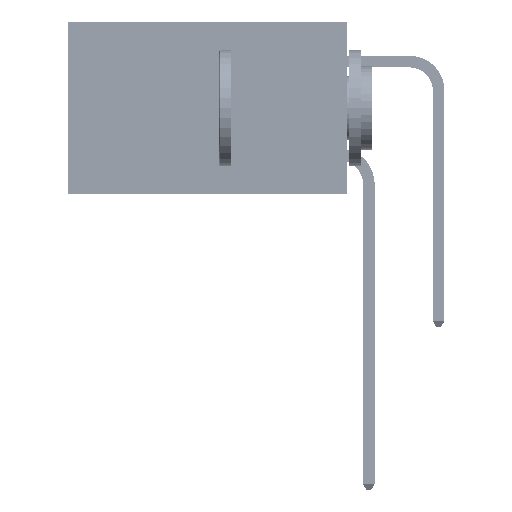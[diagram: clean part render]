
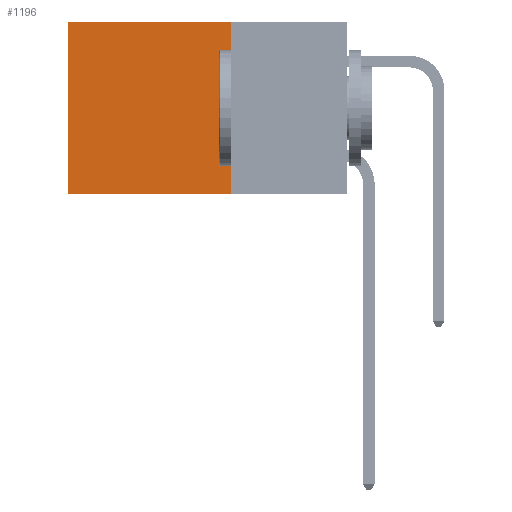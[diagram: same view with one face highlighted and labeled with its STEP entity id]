
A CAD part, left-side view. The second image highlights one B-rep face of the part: STEP entity #1196.
In plain terms, the highlighted planar face has unit normal (-1, 0, 0).
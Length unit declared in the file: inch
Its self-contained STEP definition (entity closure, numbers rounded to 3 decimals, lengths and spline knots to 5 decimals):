
#657 = FACE_OUTER_BOUND ( 'NONE', #15246, .T. ) ;
#1196 = ADVANCED_FACE ( 'NONE', ( #657 ), #12207, .F. ) ;
#1777 = VECTOR ( 'NONE', #40079, 39.37008 ) ;
#3276 = CARTESIAN_POINT ( 'NONE',  ( 0.2875, 0.6, -0.37 ) ) ;
#4918 = CARTESIAN_POINT ( 'NONE',  ( 0.2875, 0.25, 0. ) ) ;
#5480 = ORIENTED_EDGE ( 'NONE', *, *, #32674, .T. ) ;
#9277 = EDGE_CURVE ( 'NONE', #25299, #16981, #23393, .T. ) ;
#10438 = VECTOR ( 'NONE', #32113, 39.37008 ) ;
#10470 = ORIENTED_EDGE ( 'NONE', *, *, #14116, .F. ) ;
#11376 = VECTOR ( 'NONE', #34717, 39.37008 ) ;
#11385 = DIRECTION ( 'NONE',  ( 0., 0., -1. ) ) ;
#12207 = PLANE ( 'NONE',  #44484 ) ;
#13374 = VERTEX_POINT ( 'NONE', #3276 ) ;
#14008 = ORIENTED_EDGE ( 'NONE', *, *, #30318, .F. ) ;
#14116 = EDGE_CURVE ( 'NONE', #25299, #25051, #41938, .T. ) ;
#15246 = EDGE_LOOP ( 'NONE', ( #5480, #14008, #10470, #40561 ) ) ;
#15580 = CARTESIAN_POINT ( 'NONE',  ( 0.2875, 0.6, 0. ) ) ;
#16048 = DIRECTION ( 'NONE',  ( 1., 0., 0. ) ) ;
#16981 = VERTEX_POINT ( 'NONE', #37131 ) ;
#22163 = LINE ( 'NONE', #15580, #31791 ) ;
#23393 = LINE ( 'NONE', #4918, #1777 ) ;
#24009 = CARTESIAN_POINT ( 'NONE',  ( 0.2875, 0.25, -0.37 ) ) ;
#24281 = LINE ( 'NONE', #43136, #10438 ) ;
#25051 = VERTEX_POINT ( 'NONE', #24009 ) ;
#25299 = VERTEX_POINT ( 'NONE', #45358 ) ;
#30318 = EDGE_CURVE ( 'NONE', #25051, #13374, #24281, .T. ) ;
#30554 = CARTESIAN_POINT ( 'NONE',  ( 0.2875, 0.25, 0. ) ) ;
#31791 = VECTOR ( 'NONE', #11385, 39.37008 ) ;
#32113 = DIRECTION ( 'NONE',  ( 0., 1., 0. ) ) ;
#32674 = EDGE_CURVE ( 'NONE', #16981, #13374, #22163, .T. ) ;
#34717 = DIRECTION ( 'NONE',  ( 0., 0., -1. ) ) ;
#37131 = CARTESIAN_POINT ( 'NONE',  ( 0.2875, 0.6, 0. ) ) ;
#38991 = CARTESIAN_POINT ( 'NONE',  ( 0.2875, 0.25, 0. ) ) ;
#40079 = DIRECTION ( 'NONE',  ( 0., 1., 0. ) ) ;
#40561 = ORIENTED_EDGE ( 'NONE', *, *, #9277, .T. ) ;
#41938 = LINE ( 'NONE', #30554, #11376 ) ;
#42828 = DIRECTION ( 'NONE',  ( 0., 0., -1. ) ) ;
#43136 = CARTESIAN_POINT ( 'NONE',  ( 0.2875, 0.25, -0.37 ) ) ;
#44484 = AXIS2_PLACEMENT_3D ( 'NONE', #38991, #16048, #42828 ) ;
#45358 = CARTESIAN_POINT ( 'NONE',  ( 0.2875, 0.25, 0. ) ) ;
